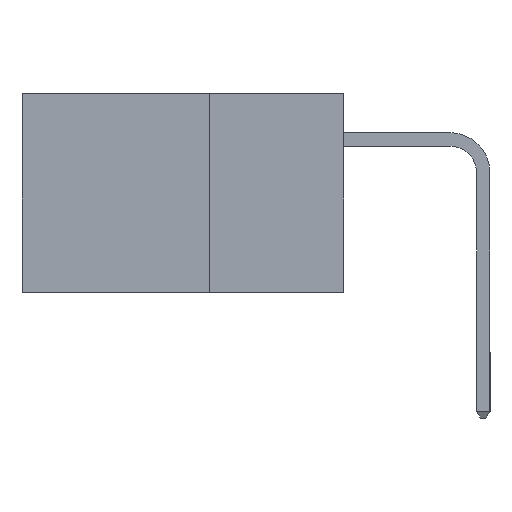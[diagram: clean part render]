
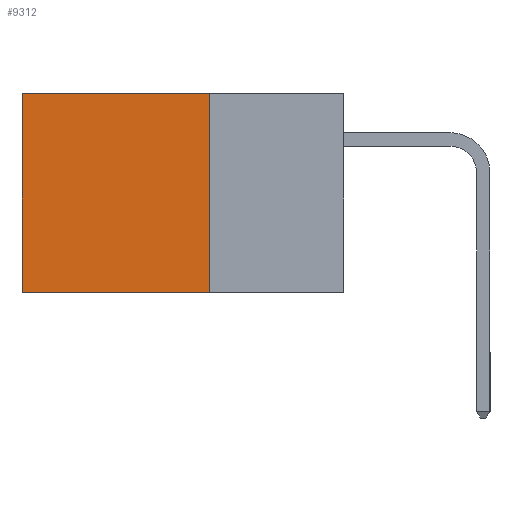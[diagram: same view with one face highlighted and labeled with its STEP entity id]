
A CAD part, left-side view. The second image highlights one B-rep face of the part: STEP entity #9312.
In plain terms, the highlighted planar face has unit normal (-1, 0, 0).
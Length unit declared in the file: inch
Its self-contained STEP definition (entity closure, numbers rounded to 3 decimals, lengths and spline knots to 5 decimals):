
#1835 = CARTESIAN_POINT ( 'NONE',  ( 0.298, 0.25, 0. ) ) ;
#2380 = VERTEX_POINT ( 'NONE', #26655 ) ;
#4813 = ORIENTED_EDGE ( 'NONE', *, *, #26879, .F. ) ;
#5242 = ORIENTED_EDGE ( 'NONE', *, *, #13000, .T. ) ;
#5473 = CARTESIAN_POINT ( 'NONE',  ( 0.298, 0.25, -0.37 ) ) ;
#5486 = LINE ( 'NONE', #5473, #21622 ) ;
#6076 = CARTESIAN_POINT ( 'NONE',  ( 0.298, 0.6, 0. ) ) ;
#6153 = DIRECTION ( 'NONE',  ( 0., 0., -1. ) ) ;
#9245 = VERTEX_POINT ( 'NONE', #17352 ) ;
#9312 = ADVANCED_FACE ( 'NONE', ( #11815 ), #17645, .F. ) ;
#10565 = VECTOR ( 'NONE', #28655, 39.37008 ) ;
#11408 = CARTESIAN_POINT ( 'NONE',  ( 0.298, 0.25, 0. ) ) ;
#11584 = VECTOR ( 'NONE', #15990, 39.37008 ) ;
#11815 = FACE_OUTER_BOUND ( 'NONE', #19089, .T. ) ;
#13000 = EDGE_CURVE ( 'NONE', #18624, #9245, #19073, .T. ) ;
#13101 = CARTESIAN_POINT ( 'NONE',  ( 0.298, 0.25, 0. ) ) ;
#13738 = CARTESIAN_POINT ( 'NONE',  ( 0.298, 0.25, 0. ) ) ;
#15990 = DIRECTION ( 'NONE',  ( 0., 0., -1. ) ) ;
#16987 = DIRECTION ( 'NONE',  ( 0., 1., 0. ) ) ;
#17352 = CARTESIAN_POINT ( 'NONE',  ( 0.298, 0.6, 0. ) ) ;
#17645 = PLANE ( 'NONE',  #26762 ) ;
#18014 = DIRECTION ( 'NONE',  ( 0., 1., 0. ) ) ;
#18386 = VECTOR ( 'NONE', #18014, 39.37008 ) ;
#18624 = VERTEX_POINT ( 'NONE', #11408 ) ;
#19073 = LINE ( 'NONE', #1835, #18386 ) ;
#19089 = EDGE_LOOP ( 'NONE', ( #28549, #22461, #4813, #5242 ) ) ;
#19903 = DIRECTION ( 'NONE',  ( 1., 0., 0. ) ) ;
#21622 = VECTOR ( 'NONE', #16987, 39.37008 ) ;
#22461 = ORIENTED_EDGE ( 'NONE', *, *, #23443, .F. ) ;
#23289 = LINE ( 'NONE', #6076, #10565 ) ;
#23443 = EDGE_CURVE ( 'NONE', #2380, #27906, #5486, .T. ) ;
#25877 = EDGE_CURVE ( 'NONE', #9245, #27906, #23289, .T. ) ;
#26655 = CARTESIAN_POINT ( 'NONE',  ( 0.298, 0.25, -0.37 ) ) ;
#26762 = AXIS2_PLACEMENT_3D ( 'NONE', #13101, #19903, #6153 ) ;
#26842 = CARTESIAN_POINT ( 'NONE',  ( 0.298, 0.6, -0.37 ) ) ;
#26879 = EDGE_CURVE ( 'NONE', #18624, #2380, #29375, .T. ) ;
#27906 = VERTEX_POINT ( 'NONE', #26842 ) ;
#28549 = ORIENTED_EDGE ( 'NONE', *, *, #25877, .T. ) ;
#28655 = DIRECTION ( 'NONE',  ( 0., 0., -1. ) ) ;
#29375 = LINE ( 'NONE', #13738, #11584 ) ;
